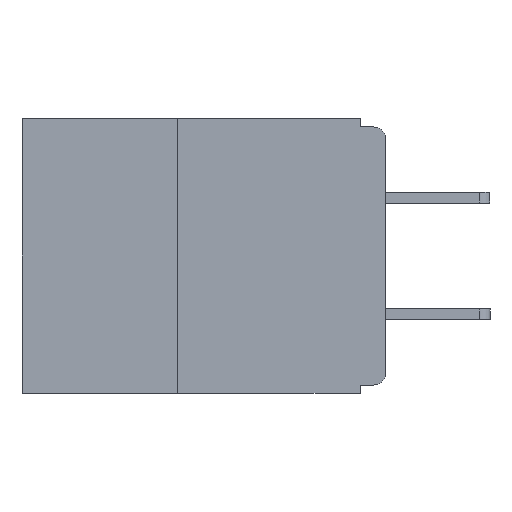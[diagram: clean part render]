
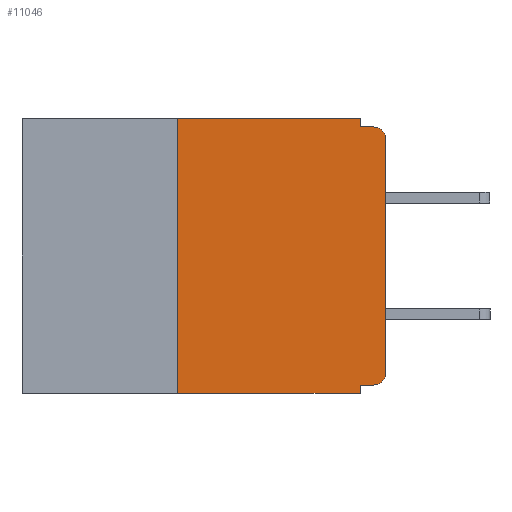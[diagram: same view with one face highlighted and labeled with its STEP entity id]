
A CAD part, left-side view. The second image highlights one B-rep face of the part: STEP entity #11046.
In plain terms, the highlighted planar face has unit normal (-1, 0, 0).
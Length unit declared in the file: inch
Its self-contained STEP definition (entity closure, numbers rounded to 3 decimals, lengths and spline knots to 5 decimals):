
#328 = CARTESIAN_POINT ( 'NONE',  ( 0., 0., 0. ) ) ;
#339 = DIRECTION ( 'NONE',  ( 0., 0., -1. ) ) ;
#358 = DIRECTION ( 'NONE',  ( -1., 0., 0. ) ) ;
#408 = CARTESIAN_POINT ( 'NONE',  ( 0., 0.015, -0.305 ) ) ;
#420 = VERTEX_POINT ( 'NONE', #2484 ) ;
#480 = ORIENTED_EDGE ( 'NONE', *, *, #10418, .T. ) ;
#530 = VECTOR ( 'NONE', #18556, 39.37008 ) ;
#543 = CARTESIAN_POINT ( 'NONE',  ( 0., 0.015, -0.32 ) ) ;
#783 = ORIENTED_EDGE ( 'NONE', *, *, #15662, .F. ) ;
#1129 = ORIENTED_EDGE ( 'NONE', *, *, #6407, .T. ) ;
#1418 = DIRECTION ( 'NONE',  ( 0., 0., -1. ) ) ;
#1873 = VECTOR ( 'NONE', #11053, 39.37008 ) ;
#2048 = DIRECTION ( 'NONE',  ( 0., -1., 0. ) ) ;
#2116 = ORIENTED_EDGE ( 'NONE', *, *, #18342, .F. ) ;
#2425 = PLANE ( 'NONE',  #17130 ) ;
#2484 = CARTESIAN_POINT ( 'NONE',  ( 0., 0.015, -0.01 ) ) ;
#2488 = DIRECTION ( 'NONE',  ( 1., 0., 0. ) ) ;
#2667 = LINE ( 'NONE', #328, #3702 ) ;
#3644 = VECTOR ( 'NONE', #17605, 39.37008 ) ;
#3702 = VECTOR ( 'NONE', #6767, 39.37008 ) ;
#3746 = EDGE_CURVE ( 'NONE', #5019, #10351, #7839, .T. ) ;
#3818 = LINE ( 'NONE', #12416, #19549 ) ;
#3935 = EDGE_CURVE ( 'NONE', #7268, #420, #4363, .T. ) ;
#4024 = LINE ( 'NONE', #11490, #8217 ) ;
#4184 = CARTESIAN_POINT ( 'NONE',  ( 0., 0., -0.025 ) ) ;
#4325 = ORIENTED_EDGE ( 'NONE', *, *, #4540, .F. ) ;
#4363 = LINE ( 'NONE', #12206, #530 ) ;
#4540 = EDGE_CURVE ( 'NONE', #19668, #16004, #18215, .T. ) ;
#4588 = CARTESIAN_POINT ( 'NONE',  ( 0., 0.031, 0. ) ) ;
#4833 = CARTESIAN_POINT ( 'NONE',  ( 0., 0.031, -0.32 ) ) ;
#5019 = VERTEX_POINT ( 'NONE', #4833 ) ;
#5293 = LINE ( 'NONE', #10515, #17481 ) ;
#5352 = DIRECTION ( 'NONE',  ( 0., 0., 1. ) ) ;
#5803 = DIRECTION ( 'NONE',  ( 0., -1., 0. ) ) ;
#5885 = CARTESIAN_POINT ( 'NONE',  ( 0., 0.25, -0.33 ) ) ;
#5917 = CARTESIAN_POINT ( 'NONE',  ( 0., 0.25, -0.33 ) ) ;
#6407 = EDGE_CURVE ( 'NONE', #10797, #8149, #17937, .T. ) ;
#6767 = DIRECTION ( 'NONE',  ( 0., 0., 1. ) ) ;
#6778 = VERTEX_POINT ( 'NONE', #4184 ) ;
#7258 = CARTESIAN_POINT ( 'NONE',  ( 0., 0.031, -0.33 ) ) ;
#7268 = VERTEX_POINT ( 'NONE', #12667 ) ;
#7578 = EDGE_CURVE ( 'NONE', #6778, #420, #9134, .T. ) ;
#7790 = DIRECTION ( 'NONE',  ( 0., 0., -1. ) ) ;
#7813 = DIRECTION ( 'NONE',  ( -1., 0., 0. ) ) ;
#7839 = LINE ( 'NONE', #18168, #3644 ) ;
#7864 = CARTESIAN_POINT ( 'NONE',  ( 0., 0.015, -0.025 ) ) ;
#8149 = VERTEX_POINT ( 'NONE', #18586 ) ;
#8217 = VECTOR ( 'NONE', #2048, 39.37008 ) ;
#9134 = CIRCLE ( 'NONE', #13612, 0.015 ) ;
#9457 = CARTESIAN_POINT ( 'NONE',  ( 0., 0., -0.32 ) ) ;
#10351 = VERTEX_POINT ( 'NONE', #7258 ) ;
#10418 = EDGE_CURVE ( 'NONE', #19668, #10351, #5293, .T. ) ;
#10423 = CARTESIAN_POINT ( 'NONE',  ( 0., 0.25, 0. ) ) ;
#10515 = CARTESIAN_POINT ( 'NONE',  ( 0., 0.437, -0.33 ) ) ;
#10797 = VERTEX_POINT ( 'NONE', #543 ) ;
#11046 = ADVANCED_FACE ( 'NONE', ( #18135 ), #2425, .F. ) ;
#11053 = DIRECTION ( 'NONE',  ( 0., 1., 0. ) ) ;
#11263 = ORIENTED_EDGE ( 'NONE', *, *, #19154, .F. ) ;
#11490 = CARTESIAN_POINT ( 'NONE',  ( 0., 0.437, 0. ) ) ;
#11928 = CARTESIAN_POINT ( 'NONE',  ( 0., 0.437, 0. ) ) ;
#12071 = AXIS2_PLACEMENT_3D ( 'NONE', #408, #358, #339 ) ;
#12206 = CARTESIAN_POINT ( 'NONE',  ( 0., 0., -0.01 ) ) ;
#12416 = CARTESIAN_POINT ( 'NONE',  ( 0., 0.031, 0. ) ) ;
#12667 = CARTESIAN_POINT ( 'NONE',  ( 0., 0.031, -0.01 ) ) ;
#12801 = EDGE_CURVE ( 'NONE', #8149, #6778, #2667, .T. ) ;
#13461 = DIRECTION ( 'NONE',  ( 0., 0., -1. ) ) ;
#13612 = AXIS2_PLACEMENT_3D ( 'NONE', #7864, #7813, #7790 ) ;
#13623 = ORIENTED_EDGE ( 'NONE', *, *, #12801, .T. ) ;
#13810 = VECTOR ( 'NONE', #5352, 39.37008 ) ;
#15033 = EDGE_LOOP ( 'NONE', ( #13623, #17101, #19112, #2116, #11263, #4325, #480, #15321, #783, #1129 ) ) ;
#15321 = ORIENTED_EDGE ( 'NONE', *, *, #3746, .F. ) ;
#15662 = EDGE_CURVE ( 'NONE', #10797, #5019, #18275, .T. ) ;
#16004 = VERTEX_POINT ( 'NONE', #10423 ) ;
#17101 = ORIENTED_EDGE ( 'NONE', *, *, #7578, .T. ) ;
#17130 = AXIS2_PLACEMENT_3D ( 'NONE', #11928, #2488, #13461 ) ;
#17481 = VECTOR ( 'NONE', #5803, 39.37008 ) ;
#17605 = DIRECTION ( 'NONE',  ( 0., 0., -1. ) ) ;
#17937 = CIRCLE ( 'NONE', #12071, 0.015 ) ;
#18135 = FACE_OUTER_BOUND ( 'NONE', #15033, .T. ) ;
#18168 = CARTESIAN_POINT ( 'NONE',  ( 0., 0.031, -0.33 ) ) ;
#18215 = LINE ( 'NONE', #5885, #13810 ) ;
#18275 = LINE ( 'NONE', #9457, #1873 ) ;
#18342 = EDGE_CURVE ( 'NONE', #19754, #7268, #3818, .T. ) ;
#18556 = DIRECTION ( 'NONE',  ( 0., -1., 0. ) ) ;
#18586 = CARTESIAN_POINT ( 'NONE',  ( 0., 0., -0.305 ) ) ;
#19112 = ORIENTED_EDGE ( 'NONE', *, *, #3935, .F. ) ;
#19154 = EDGE_CURVE ( 'NONE', #16004, #19754, #4024, .T. ) ;
#19549 = VECTOR ( 'NONE', #1418, 39.37008 ) ;
#19668 = VERTEX_POINT ( 'NONE', #5917 ) ;
#19754 = VERTEX_POINT ( 'NONE', #4588 ) ;
